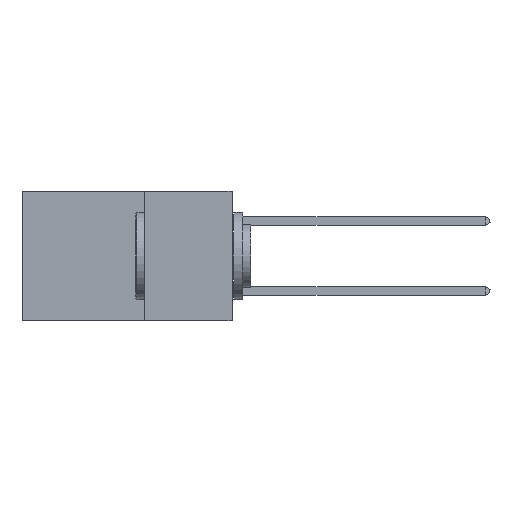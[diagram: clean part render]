
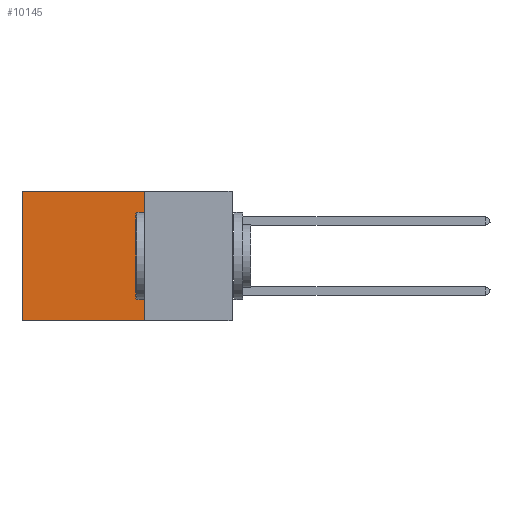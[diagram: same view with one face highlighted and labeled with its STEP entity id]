
A CAD part, left-side view. The second image highlights one B-rep face of the part: STEP entity #10145.
In plain terms, the highlighted planar face has unit normal (-1, 0, 0).
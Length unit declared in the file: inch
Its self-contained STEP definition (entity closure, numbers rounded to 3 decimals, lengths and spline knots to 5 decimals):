
#490 = EDGE_CURVE ( 'NONE', #23881, #16842, #16454, .T. ) ;
#1886 = VECTOR ( 'NONE', #18133, 39.37008 ) ;
#3244 = CARTESIAN_POINT ( 'NONE',  ( 0.2875, 0.25, 0. ) ) ;
#3774 = EDGE_CURVE ( 'NONE', #24501, #19174, #7995, .T. ) ;
#4076 = CARTESIAN_POINT ( 'NONE',  ( 0.2875, 0.25, 0. ) ) ;
#4664 = VECTOR ( 'NONE', #20289, 39.37008 ) ;
#4854 = CARTESIAN_POINT ( 'NONE',  ( 0.2875, 0.25, -0.37 ) ) ;
#4982 = CARTESIAN_POINT ( 'NONE',  ( 0.2875, 0.25, -0.37 ) ) ;
#5604 = DIRECTION ( 'NONE',  ( 1., 0., 0. ) ) ;
#5793 = FACE_OUTER_BOUND ( 'NONE', #19034, .T. ) ;
#6206 = CARTESIAN_POINT ( 'NONE',  ( 0.2875, 0.6, -0.37 ) ) ;
#6420 = LINE ( 'NONE', #4854, #1886 ) ;
#7307 = VECTOR ( 'NONE', #26279, 39.37008 ) ;
#7729 = DIRECTION ( 'NONE',  ( 0., 1., 0. ) ) ;
#7995 = LINE ( 'NONE', #13130, #7307 ) ;
#8223 = AXIS2_PLACEMENT_3D ( 'NONE', #12186, #5604, #21102 ) ;
#10145 = ADVANCED_FACE ( 'NONE', ( #5793 ), #18887, .F. ) ;
#10509 = CARTESIAN_POINT ( 'NONE',  ( 0.2875, 0.25, 0. ) ) ;
#12186 = CARTESIAN_POINT ( 'NONE',  ( 0.2875, 0.25, 0. ) ) ;
#13130 = CARTESIAN_POINT ( 'NONE',  ( 0.2875, 0.6, 0. ) ) ;
#13621 = VECTOR ( 'NONE', #7729, 39.37008 ) ;
#14121 = ORIENTED_EDGE ( 'NONE', *, *, #17414, .F. ) ;
#14858 = ORIENTED_EDGE ( 'NONE', *, *, #22230, .T. ) ;
#15922 = CARTESIAN_POINT ( 'NONE',  ( 0.2875, 0.6, 0. ) ) ;
#16454 = LINE ( 'NONE', #4076, #4664 ) ;
#16842 = VERTEX_POINT ( 'NONE', #4982 ) ;
#17414 = EDGE_CURVE ( 'NONE', #16842, #19174, #6420, .T. ) ;
#18133 = DIRECTION ( 'NONE',  ( 0., 1., 0. ) ) ;
#18887 = PLANE ( 'NONE',  #8223 ) ;
#19034 = EDGE_LOOP ( 'NONE', ( #22995, #14121, #20155, #14858 ) ) ;
#19174 = VERTEX_POINT ( 'NONE', #6206 ) ;
#20155 = ORIENTED_EDGE ( 'NONE', *, *, #490, .F. ) ;
#20289 = DIRECTION ( 'NONE',  ( 0., 0., -1. ) ) ;
#21102 = DIRECTION ( 'NONE',  ( 0., 0., -1. ) ) ;
#22230 = EDGE_CURVE ( 'NONE', #23881, #24501, #24659, .T. ) ;
#22995 = ORIENTED_EDGE ( 'NONE', *, *, #3774, .T. ) ;
#23881 = VERTEX_POINT ( 'NONE', #10509 ) ;
#24501 = VERTEX_POINT ( 'NONE', #15922 ) ;
#24659 = LINE ( 'NONE', #3244, #13621 ) ;
#26279 = DIRECTION ( 'NONE',  ( 0., 0., -1. ) ) ;
